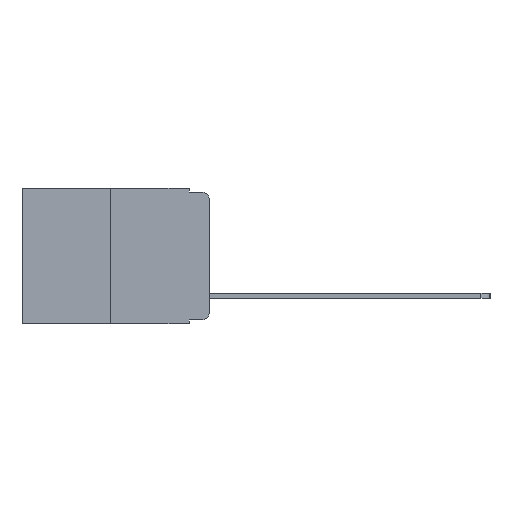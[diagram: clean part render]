
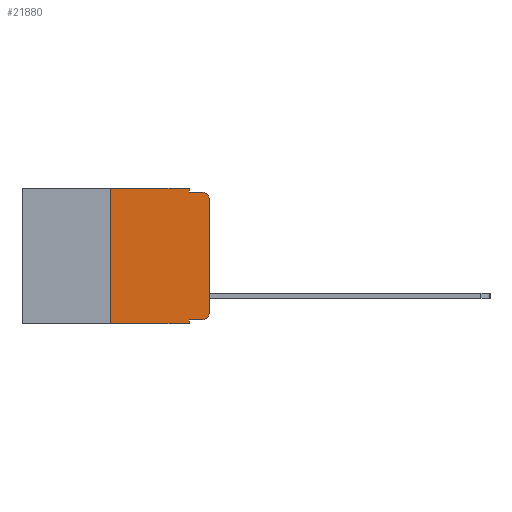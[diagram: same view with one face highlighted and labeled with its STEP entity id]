
A CAD part, left-side view. The second image highlights one B-rep face of the part: STEP entity #21880.
In plain terms, the highlighted planar face has unit normal (-1, 0, 0).
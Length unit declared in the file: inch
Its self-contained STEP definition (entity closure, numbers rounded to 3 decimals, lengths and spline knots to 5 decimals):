
#172 = ORIENTED_EDGE ( 'NONE', *, *, #10502, .T. ) ;
#345 = VERTEX_POINT ( 'NONE', #20315 ) ;
#467 = DIRECTION ( 'NONE',  ( 0., -1., 0. ) ) ;
#665 = VECTOR ( 'NONE', #16083, 39.37008 ) ;
#684 = CARTESIAN_POINT ( 'NONE',  ( 0., 0.02, -0.313 ) ) ;
#891 = VECTOR ( 'NONE', #9544, 39.37008 ) ;
#1276 = LINE ( 'NONE', #10211, #21418 ) ;
#1301 = DIRECTION ( 'NONE',  ( 1., 0., 0. ) ) ;
#1480 = EDGE_CURVE ( 'NONE', #21696, #24236, #21892, .T. ) ;
#2715 = DIRECTION ( 'NONE',  ( 0., 0., -1. ) ) ;
#3241 = CARTESIAN_POINT ( 'NONE',  ( 0., 0.051, -0.343 ) ) ;
#3931 = EDGE_CURVE ( 'NONE', #21696, #24950, #1276, .T. ) ;
#4325 = VERTEX_POINT ( 'NONE', #15569 ) ;
#4331 = ORIENTED_EDGE ( 'NONE', *, *, #7987, .F. ) ;
#4353 = CARTESIAN_POINT ( 'NONE',  ( 0., 0., 0. ) ) ;
#4394 = CARTESIAN_POINT ( 'NONE',  ( 0., 0.473, 0. ) ) ;
#5967 = CARTESIAN_POINT ( 'NONE',  ( 0., 0.02, -0.333 ) ) ;
#6094 = DIRECTION ( 'NONE',  ( 0., 0., -1. ) ) ;
#6366 = EDGE_CURVE ( 'NONE', #24950, #345, #24780, .T. ) ;
#6557 = ORIENTED_EDGE ( 'NONE', *, *, #22553, .F. ) ;
#6754 = CARTESIAN_POINT ( 'NONE',  ( 0., 0.25, -0.343 ) ) ;
#6793 = CARTESIAN_POINT ( 'NONE',  ( 0., 0.051, -0.01 ) ) ;
#7273 = FACE_OUTER_BOUND ( 'NONE', #9714, .T. ) ;
#7549 = CARTESIAN_POINT ( 'NONE',  ( 0., 0.051, 0. ) ) ;
#7987 = EDGE_CURVE ( 'NONE', #16863, #24236, #19451, .T. ) ;
#8043 = CIRCLE ( 'NONE', #14900, 0.02 ) ;
#8209 = VERTEX_POINT ( 'NONE', #6793 ) ;
#8226 = DIRECTION ( 'NONE',  ( 0., 0., 1. ) ) ;
#8616 = DIRECTION ( 'NONE',  ( 0., -1., 0. ) ) ;
#9160 = EDGE_CURVE ( 'NONE', #16863, #23818, #13922, .T. ) ;
#9544 = DIRECTION ( 'NONE',  ( 0., 0., -1. ) ) ;
#9629 = ORIENTED_EDGE ( 'NONE', *, *, #9160, .T. ) ;
#9714 = EDGE_LOOP ( 'NONE', ( #10580, #11194, #21281, #6557, #18059, #23025, #14204, #4331, #9629, #172 ) ) ;
#10211 = CARTESIAN_POINT ( 'NONE',  ( 0., 0.25, 0. ) ) ;
#10502 = EDGE_CURVE ( 'NONE', #23818, #17243, #8043, .T. ) ;
#10536 = DIRECTION ( 'NONE',  ( -1., 0., 0. ) ) ;
#10580 = ORIENTED_EDGE ( 'NONE', *, *, #21130, .T. ) ;
#11142 = EDGE_CURVE ( 'NONE', #8209, #14838, #17362, .T. ) ;
#11194 = ORIENTED_EDGE ( 'NONE', *, *, #15595, .T. ) ;
#11313 = CARTESIAN_POINT ( 'NONE',  ( 0., 0.473, 0. ) ) ;
#11806 = VECTOR ( 'NONE', #23839, 39.37008 ) ;
#11993 = CARTESIAN_POINT ( 'NONE',  ( 0., 0., -0.313 ) ) ;
#12338 = VECTOR ( 'NONE', #467, 39.37008 ) ;
#13846 = VECTOR ( 'NONE', #6094, 39.37008 ) ;
#13863 = CARTESIAN_POINT ( 'NONE',  ( 0., 0.02, -0.01 ) ) ;
#13922 = LINE ( 'NONE', #23845, #23337 ) ;
#14204 = ORIENTED_EDGE ( 'NONE', *, *, #1480, .T. ) ;
#14387 = CARTESIAN_POINT ( 'NONE',  ( 0., 0.051, -0.01 ) ) ;
#14574 = DIRECTION ( 'NONE',  ( -1., 0., 0. ) ) ;
#14838 = VERTEX_POINT ( 'NONE', #13863 ) ;
#14900 = AXIS2_PLACEMENT_3D ( 'NONE', #684, #14574, #2715 ) ;
#15156 = DIRECTION ( 'NONE',  ( 0., 0., -1. ) ) ;
#15564 = AXIS2_PLACEMENT_3D ( 'NONE', #11313, #1301, #15156 ) ;
#15569 = CARTESIAN_POINT ( 'NONE',  ( 0., 0., -0.03 ) ) ;
#15595 = EDGE_CURVE ( 'NONE', #4325, #14838, #24263, .T. ) ;
#15800 = CARTESIAN_POINT ( 'NONE',  ( 0., 0.051, 0. ) ) ;
#15831 = LINE ( 'NONE', #4353, #665 ) ;
#16083 = DIRECTION ( 'NONE',  ( 0., 0., 1. ) ) ;
#16123 = DIRECTION ( 'NONE',  ( 0., -1., 0. ) ) ;
#16577 = CARTESIAN_POINT ( 'NONE',  ( 0., 0.051, -0.333 ) ) ;
#16627 = LINE ( 'NONE', #7549, #891 ) ;
#16863 = VERTEX_POINT ( 'NONE', #16577 ) ;
#17243 = VERTEX_POINT ( 'NONE', #11993 ) ;
#17362 = LINE ( 'NONE', #14387, #12338 ) ;
#18059 = ORIENTED_EDGE ( 'NONE', *, *, #6366, .F. ) ;
#19451 = LINE ( 'NONE', #15800, #13846 ) ;
#19582 = AXIS2_PLACEMENT_3D ( 'NONE', #21915, #10536, #23781 ) ;
#19839 = VECTOR ( 'NONE', #16123, 39.37008 ) ;
#20315 = CARTESIAN_POINT ( 'NONE',  ( 0., 0.051, 0. ) ) ;
#21130 = EDGE_CURVE ( 'NONE', #17243, #4325, #15831, .T. ) ;
#21281 = ORIENTED_EDGE ( 'NONE', *, *, #11142, .F. ) ;
#21418 = VECTOR ( 'NONE', #8226, 39.37008 ) ;
#21696 = VERTEX_POINT ( 'NONE', #6754 ) ;
#21880 = ADVANCED_FACE ( 'NONE', ( #7273 ), #24507, .F. ) ;
#21892 = LINE ( 'NONE', #24232, #11806 ) ;
#21915 = CARTESIAN_POINT ( 'NONE',  ( 0., 0.02, -0.03 ) ) ;
#22553 = EDGE_CURVE ( 'NONE', #345, #8209, #16627, .T. ) ;
#22857 = CARTESIAN_POINT ( 'NONE',  ( 0., 0.25, 0. ) ) ;
#23025 = ORIENTED_EDGE ( 'NONE', *, *, #3931, .F. ) ;
#23337 = VECTOR ( 'NONE', #8616, 39.37008 ) ;
#23781 = DIRECTION ( 'NONE',  ( 0., 0., -1. ) ) ;
#23818 = VERTEX_POINT ( 'NONE', #5967 ) ;
#23839 = DIRECTION ( 'NONE',  ( 0., -1., 0. ) ) ;
#23845 = CARTESIAN_POINT ( 'NONE',  ( 0., 0.051, -0.333 ) ) ;
#24232 = CARTESIAN_POINT ( 'NONE',  ( 0., 0.473, -0.343 ) ) ;
#24236 = VERTEX_POINT ( 'NONE', #3241 ) ;
#24263 = CIRCLE ( 'NONE', #19582, 0.02 ) ;
#24507 = PLANE ( 'NONE',  #15564 ) ;
#24780 = LINE ( 'NONE', #4394, #19839 ) ;
#24950 = VERTEX_POINT ( 'NONE', #22857 ) ;
